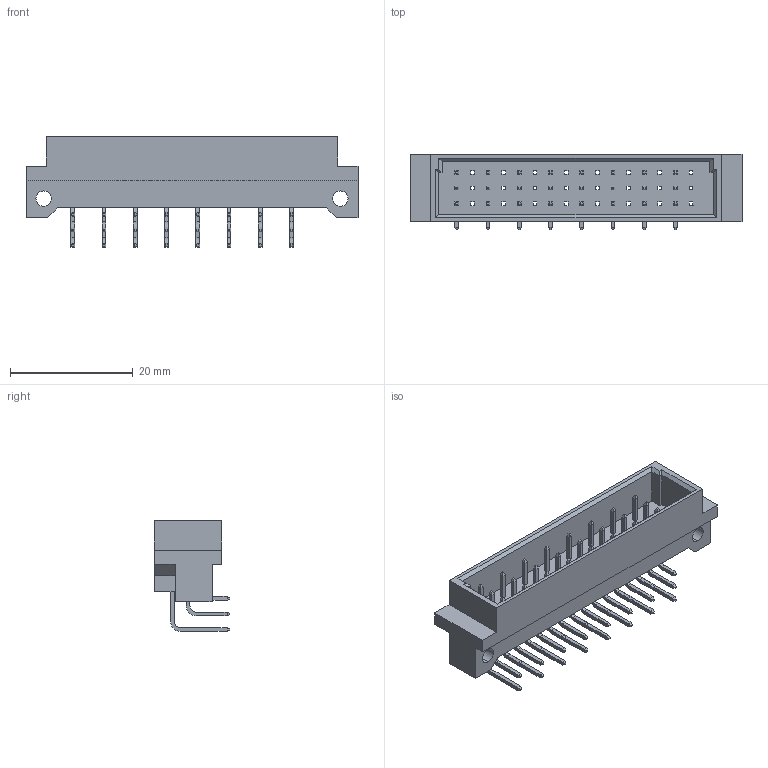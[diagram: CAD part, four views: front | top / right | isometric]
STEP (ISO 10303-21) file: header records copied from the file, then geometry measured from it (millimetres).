
FILE_DESCRIPTION (( 'STEP AP214' ), '1' );
FILE_NAME ('495-024-660-322.STEP', '2020-08-12T15:21:42', ( '' ), ( '' ), 'SwSTEP 2.0', 'SolidWorks 2020', '' );
FILE_SCHEMA (( 'AUTOMOTIVE_DESIGN' ));
Length unit declared in the file: millimetre
Products named in the file (5): 495-024-660-322; 495-290-2; 495 Part_48; 495-290-1; 495-290-3
Assembly tree (25 placements, depth 2):
  495-024-660-322
    495 Part_48
    495-290-1  x8
    495-290-2  x8
    495-290-3  x8
Bounding box: 54 x 12.27 x 18.05 mm (x, y, z)
Volume: 3622.4 mm3; surface area: 5112.5 mm2
Topology: 25 solids, 25 shells, 674 faces, 1664 edges, 1042 vertices
Faces by surface type: plane 622, cylinder 52
Entity records: 9822 total; most frequent: CARTESIAN_POINT 1686, ORIENTED_EDGE 1648, DIRECTION 1492, EDGE_CURVE 824, LINE 804, VECTOR 804, VERTEX_POINT 538, EDGE_LOOP 398
